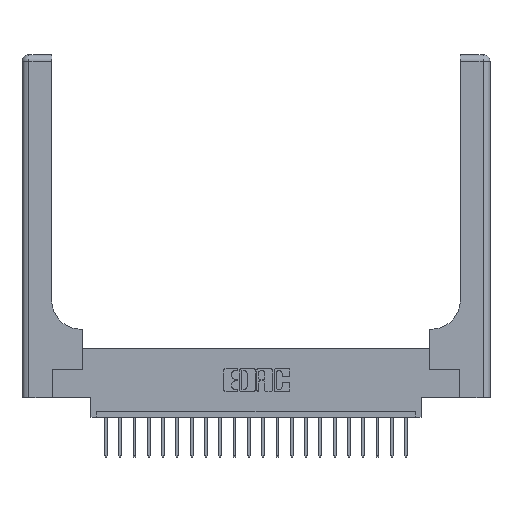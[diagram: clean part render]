
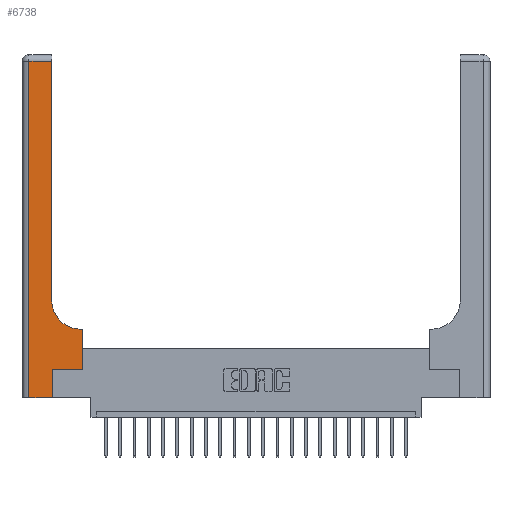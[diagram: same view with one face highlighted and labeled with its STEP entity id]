
A CAD part, top view. The second image highlights one B-rep face of the part: STEP entity #6738.
In plain terms, the highlighted planar face has unit normal (0, 0, 1).
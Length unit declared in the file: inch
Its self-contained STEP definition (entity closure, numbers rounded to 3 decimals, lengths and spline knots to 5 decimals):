
#32 = CARTESIAN_POINT ( 'NONE',  ( 0.265, 0., 0.37 ) ) ;
#955 = AXIS2_PLACEMENT_3D ( 'NONE', #15775, #20723, #7361 ) ;
#1037 = EDGE_CURVE ( 'NONE', #20028, #8023, #21637, .T. ) ;
#1064 = EDGE_CURVE ( 'NONE', #1665, #16403, #18441, .T. ) ;
#1665 = VERTEX_POINT ( 'NONE', #17231 ) ;
#2201 = ORIENTED_EDGE ( 'NONE', *, *, #12264, .T. ) ;
#3082 = DIRECTION ( 'NONE',  ( 1., 0., 0. ) ) ;
#3144 = ORIENTED_EDGE ( 'NONE', *, *, #20814, .T. ) ;
#3243 = DIRECTION ( 'NONE',  ( -1., 0., 0. ) ) ;
#3412 = EDGE_LOOP ( 'NONE', ( #3144, #6668, #2201, #18059, #19766, #15810, #18083, #7855, #4141 ) ) ;
#3593 = VECTOR ( 'NONE', #6295, 39.37008 ) ;
#4093 = VECTOR ( 'NONE', #18962, 39.37008 ) ;
#4141 = ORIENTED_EDGE ( 'NONE', *, *, #6267, .T. ) ;
#4268 = CARTESIAN_POINT ( 'NONE',  ( 0.528, 0.25, 0.37 ) ) ;
#4383 = CARTESIAN_POINT ( 'NONE',  ( 0.26, 2.94, 0.37 ) ) ;
#4751 = CARTESIAN_POINT ( 'NONE',  ( 0.51, 0.85, 0.37 ) ) ;
#5035 = CARTESIAN_POINT ( 'NONE',  ( 0.265, 0.25, 0.37 ) ) ;
#5061 = DIRECTION ( 'NONE',  ( 0., 1., 0. ) ) ;
#6081 = EDGE_CURVE ( 'NONE', #20923, #20028, #17728, .T. ) ;
#6267 = EDGE_CURVE ( 'NONE', #16403, #16893, #16139, .T. ) ;
#6295 = DIRECTION ( 'NONE',  ( 0., -1., 0. ) ) ;
#6668 = ORIENTED_EDGE ( 'NONE', *, *, #6683, .T. ) ;
#6683 = EDGE_CURVE ( 'NONE', #16662, #21059, #10112, .T. ) ;
#6705 = EDGE_CURVE ( 'NONE', #11514, #1665, #15580, .T. ) ;
#6738 = ADVANCED_FACE ( 'NONE', ( #6933 ), #7303, .F. ) ;
#6878 = DIRECTION ( 'NONE',  ( 0., 1., 0. ) ) ;
#6933 = FACE_OUTER_BOUND ( 'NONE', #3412, .T. ) ;
#7303 = PLANE ( 'NONE',  #955 ) ;
#7361 = DIRECTION ( 'NONE',  ( -1., 0., 0. ) ) ;
#7509 = DIRECTION ( 'NONE',  ( 0., 1., 0. ) ) ;
#7855 = ORIENTED_EDGE ( 'NONE', *, *, #1064, .T. ) ;
#8023 = VERTEX_POINT ( 'NONE', #14039 ) ;
#8742 = VECTOR ( 'NONE', #3243, 39.37008 ) ;
#10033 = CARTESIAN_POINT ( 'NONE',  ( 0.51, 0.6, 0.37 ) ) ;
#10089 = VECTOR ( 'NONE', #7509, 39.37008 ) ;
#10112 = LINE ( 'NONE', #19232, #17452 ) ;
#10414 = CARTESIAN_POINT ( 'NONE',  ( 0.06, 0., 0.37 ) ) ;
#10594 = CARTESIAN_POINT ( 'NONE',  ( 0.528, 0.25, 0.37 ) ) ;
#10746 = DIRECTION ( 'NONE',  ( -1., 0., 0. ) ) ;
#11212 = CARTESIAN_POINT ( 'NONE',  ( 0.06, 2.94, 0.37 ) ) ;
#11481 = CARTESIAN_POINT ( 'NONE',  ( 0.265, 0., 0.37 ) ) ;
#11514 = VERTEX_POINT ( 'NONE', #4268 ) ;
#11678 = CARTESIAN_POINT ( 'NONE',  ( 0.26, 0.85, 0.37 ) ) ;
#12264 = EDGE_CURVE ( 'NONE', #21059, #20923, #13292, .T. ) ;
#13292 = LINE ( 'NONE', #16410, #3593 ) ;
#13907 = CARTESIAN_POINT ( 'NONE',  ( 0., 0., 0.37 ) ) ;
#14039 = CARTESIAN_POINT ( 'NONE',  ( 0.265, 0.25, 0.37 ) ) ;
#14185 = VECTOR ( 'NONE', #5061, 39.37008 ) ;
#14472 = LINE ( 'NONE', #18267, #14185 ) ;
#15463 = VECTOR ( 'NONE', #18521, 39.37008 ) ;
#15580 = LINE ( 'NONE', #10594, #10089 ) ;
#15775 = CARTESIAN_POINT ( 'NONE',  ( 0., 3., 0.37 ) ) ;
#15810 = ORIENTED_EDGE ( 'NONE', *, *, #21435, .T. ) ;
#16092 = AXIS2_PLACEMENT_3D ( 'NONE', #4751, #17873, #3082 ) ;
#16139 = CIRCLE ( 'NONE', #16092, 0.25 ) ;
#16366 = VECTOR ( 'NONE', #6878, 39.37008 ) ;
#16403 = VERTEX_POINT ( 'NONE', #10033 ) ;
#16410 = CARTESIAN_POINT ( 'NONE',  ( 0.06, 3., 0.37 ) ) ;
#16662 = VERTEX_POINT ( 'NONE', #4383 ) ;
#16893 = VERTEX_POINT ( 'NONE', #11678 ) ;
#17231 = CARTESIAN_POINT ( 'NONE',  ( 0.528, 0.6, 0.37 ) ) ;
#17452 = VECTOR ( 'NONE', #10746, 39.37008 ) ;
#17728 = LINE ( 'NONE', #13907, #4093 ) ;
#17873 = DIRECTION ( 'NONE',  ( 0., 0., -1. ) ) ;
#18059 = ORIENTED_EDGE ( 'NONE', *, *, #6081, .T. ) ;
#18083 = ORIENTED_EDGE ( 'NONE', *, *, #6705, .T. ) ;
#18267 = CARTESIAN_POINT ( 'NONE',  ( 0.26, 3., 0.37 ) ) ;
#18441 = LINE ( 'NONE', #18597, #8742 ) ;
#18521 = DIRECTION ( 'NONE',  ( 1., 0., 0. ) ) ;
#18597 = CARTESIAN_POINT ( 'NONE',  ( 0.26, 0.6, 0.37 ) ) ;
#18962 = DIRECTION ( 'NONE',  ( 1., 0., 0. ) ) ;
#19232 = CARTESIAN_POINT ( 'NONE',  ( 0., 2.94, 0.37 ) ) ;
#19766 = ORIENTED_EDGE ( 'NONE', *, *, #1037, .T. ) ;
#20028 = VERTEX_POINT ( 'NONE', #11481 ) ;
#20723 = DIRECTION ( 'NONE',  ( 0., 0., -1. ) ) ;
#20814 = EDGE_CURVE ( 'NONE', #16893, #16662, #14472, .T. ) ;
#20923 = VERTEX_POINT ( 'NONE', #10414 ) ;
#21007 = LINE ( 'NONE', #5035, #15463 ) ;
#21059 = VERTEX_POINT ( 'NONE', #11212 ) ;
#21435 = EDGE_CURVE ( 'NONE', #8023, #11514, #21007, .T. ) ;
#21637 = LINE ( 'NONE', #32, #16366 ) ;
